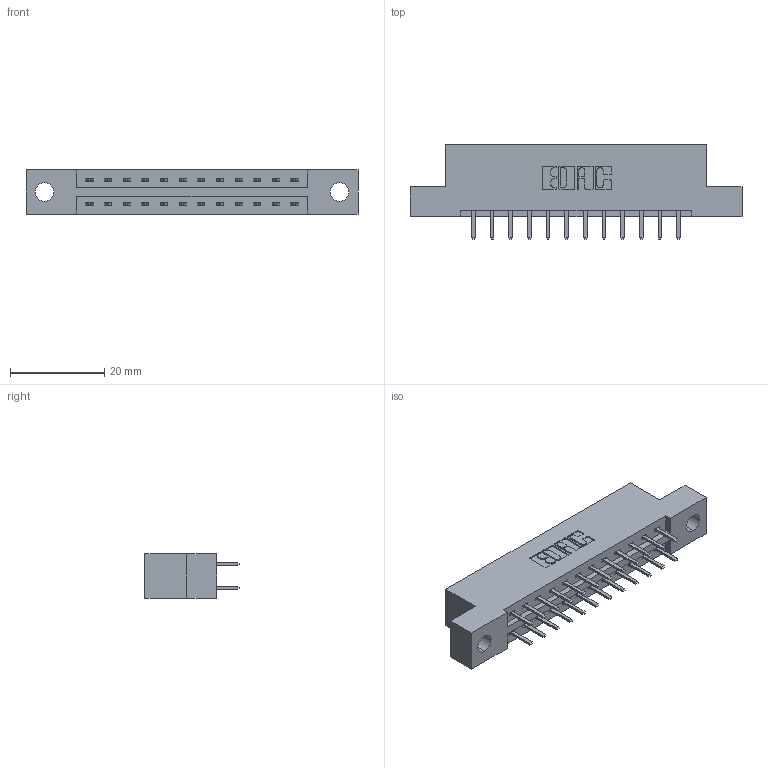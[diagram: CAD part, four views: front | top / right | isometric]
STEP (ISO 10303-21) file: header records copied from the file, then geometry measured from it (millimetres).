
FILE_DESCRIPTION (( 'STEP AP203' ), '1' );
FILE_NAME ('337-024-520-204.STEP', '2018-08-05T18:23:33', ( '' ), ( '' ), 'SwSTEP 2.0', 'SolidWorks 2016', '' );
FILE_SCHEMA (( 'CONFIG_CONTROL_DESIGN' ));
Length unit declared in the file: inch
Products named in the file (3): 337-024-520-204; 337 Part_Flush Mounting Lugs - 0.156 Dia-TH; 345-292-001_345-293-120
Assembly tree (25 placements, depth 2):
  337-024-520-204
    337 Part_Flush Mounting Lugs - 0.156 Dia-TH
    345-292-001_345-293-120  x24
Bounding box: 70.56 x 20.02 x 9.4 mm (x, y, z)
Volume: 6938.6 mm3; surface area: 7319.9 mm2
Topology: 25 solids, 25 shells, 1506 faces, 4367 edges, 2846 vertices
Faces by surface type: plane 1030, cylinder 476
Entity records: 13301 total; most frequent: CARTESIAN_POINT 2278, ORIENTED_EDGE 2202, DIRECTION 1981, EDGE_CURVE 1101, LINE 969, VECTOR 969, VERTEX_POINT 730, AXIS2_PLACEMENT_3D 506
